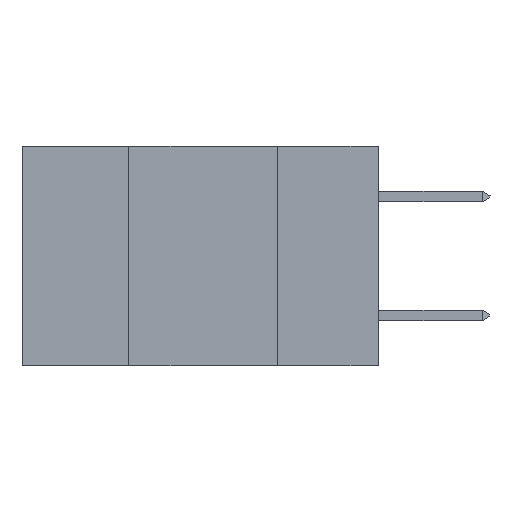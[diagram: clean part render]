
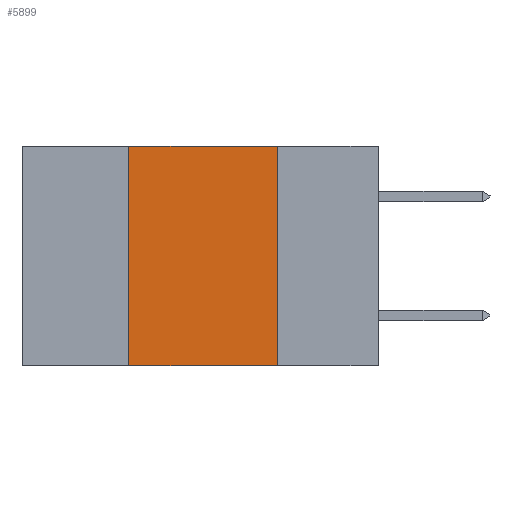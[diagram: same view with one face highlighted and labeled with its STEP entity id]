
A CAD part, left-side view. The second image highlights one B-rep face of the part: STEP entity #5899.
In plain terms, the highlighted planar face has unit normal (-1, 0, 0).
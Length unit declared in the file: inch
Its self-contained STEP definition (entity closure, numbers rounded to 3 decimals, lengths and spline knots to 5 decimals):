
#422 = VERTEX_POINT ( 'NONE', #6426 ) ;
#591 = VERTEX_POINT ( 'NONE', #5825 ) ;
#596 = DIRECTION ( 'NONE',  ( 0., -1., 0. ) ) ;
#741 = AXIS2_PLACEMENT_3D ( 'NONE', #3711, #2152, #4725 ) ;
#848 = EDGE_CURVE ( 'NONE', #422, #10124, #2992, .T. ) ;
#940 = DIRECTION ( 'NONE',  ( 0., 0., -1. ) ) ;
#1077 = ORIENTED_EDGE ( 'NONE', *, *, #2555, .F. ) ;
#1410 = DIRECTION ( 'NONE',  ( 0., 0., 1. ) ) ;
#1636 = ORIENTED_EDGE ( 'NONE', *, *, #4044, .T. ) ;
#2152 = DIRECTION ( 'NONE',  ( 1., 0., 0. ) ) ;
#2555 = EDGE_CURVE ( 'NONE', #3512, #422, #3964, .T. ) ;
#2615 = CARTESIAN_POINT ( 'NONE',  ( 0., 0.6, -0.37 ) ) ;
#2992 = LINE ( 'NONE', #7210, #8237 ) ;
#3512 = VERTEX_POINT ( 'NONE', #9426 ) ;
#3711 = CARTESIAN_POINT ( 'NONE',  ( 0., 0.6, 0. ) ) ;
#3964 = LINE ( 'NONE', #7356, #10324 ) ;
#4044 = EDGE_CURVE ( 'NONE', #3512, #591, #5339, .T. ) ;
#4265 = CARTESIAN_POINT ( 'NONE',  ( 0., 0.17, -0.37 ) ) ;
#4319 = ORIENTED_EDGE ( 'NONE', *, *, #5728, .F. ) ;
#4725 = DIRECTION ( 'NONE',  ( 0., 0., -1. ) ) ;
#5111 = LINE ( 'NONE', #4265, #8543 ) ;
#5339 = LINE ( 'NONE', #2615, #6280 ) ;
#5728 = EDGE_CURVE ( 'NONE', #10124, #591, #5111, .T. ) ;
#5825 = CARTESIAN_POINT ( 'NONE',  ( 0., 0.17, -0.37 ) ) ;
#5899 = ADVANCED_FACE ( 'NONE', ( #6365 ), #8101, .F. ) ;
#5958 = ORIENTED_EDGE ( 'NONE', *, *, #848, .F. ) ;
#5962 = EDGE_LOOP ( 'NONE', ( #4319, #5958, #1077, #1636 ) ) ;
#6280 = VECTOR ( 'NONE', #8621, 39.37008 ) ;
#6365 = FACE_OUTER_BOUND ( 'NONE', #5962, .T. ) ;
#6426 = CARTESIAN_POINT ( 'NONE',  ( 0., 0.42, 0. ) ) ;
#7210 = CARTESIAN_POINT ( 'NONE',  ( 0., 0.6, 0. ) ) ;
#7356 = CARTESIAN_POINT ( 'NONE',  ( 0., 0.42, -0.37 ) ) ;
#8101 = PLANE ( 'NONE',  #741 ) ;
#8237 = VECTOR ( 'NONE', #596, 39.37008 ) ;
#8543 = VECTOR ( 'NONE', #940, 39.37008 ) ;
#8587 = CARTESIAN_POINT ( 'NONE',  ( 0., 0.17, 0. ) ) ;
#8621 = DIRECTION ( 'NONE',  ( 0., -1., 0. ) ) ;
#9426 = CARTESIAN_POINT ( 'NONE',  ( 0., 0.42, -0.37 ) ) ;
#10124 = VERTEX_POINT ( 'NONE', #8587 ) ;
#10324 = VECTOR ( 'NONE', #1410, 39.37008 ) ;
